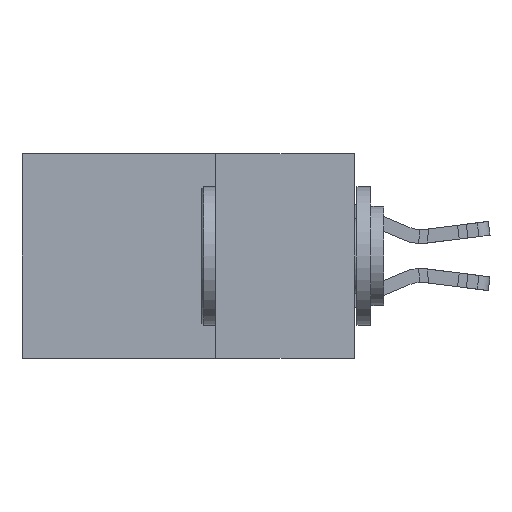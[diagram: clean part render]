
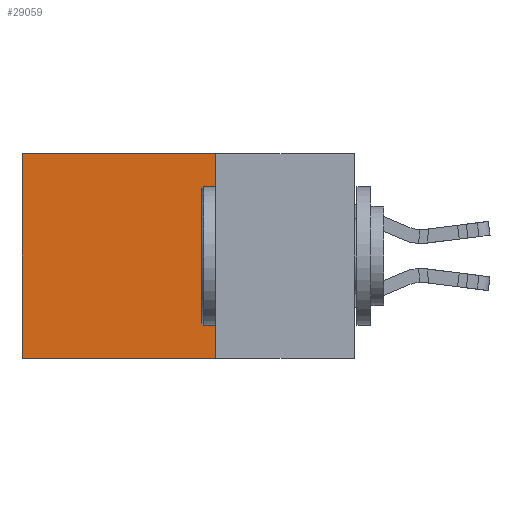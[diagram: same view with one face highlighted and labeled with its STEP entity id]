
A CAD part, left-side view. The second image highlights one B-rep face of the part: STEP entity #29059.
In plain terms, the highlighted planar face has unit normal (-1, 0, 0).
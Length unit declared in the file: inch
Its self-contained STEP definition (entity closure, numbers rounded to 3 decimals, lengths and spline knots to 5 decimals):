
#781 = CARTESIAN_POINT ( 'NONE',  ( 0.298, 0.25, 0. ) ) ;
#1526 = CARTESIAN_POINT ( 'NONE',  ( 0.298, 0.6, -0.37 ) ) ;
#2129 = DIRECTION ( 'NONE',  ( 0., 0., -1. ) ) ;
#2364 = CARTESIAN_POINT ( 'NONE',  ( 0.298, 0.6, 0. ) ) ;
#2925 = VERTEX_POINT ( 'NONE', #2364 ) ;
#3023 = VECTOR ( 'NONE', #2129, 39.37008 ) ;
#3134 = DIRECTION ( 'NONE',  ( 0., 0., -1. ) ) ;
#3246 = EDGE_LOOP ( 'NONE', ( #29673, #17705, #14978, #15695 ) ) ;
#3385 = DIRECTION ( 'NONE',  ( 0., 1., 0. ) ) ;
#3752 = EDGE_CURVE ( 'NONE', #8334, #28093, #27496, .T. ) ;
#4683 = EDGE_CURVE ( 'NONE', #2925, #28093, #22085, .T. ) ;
#4702 = CARTESIAN_POINT ( 'NONE',  ( 0.298, 0.25, 0. ) ) ;
#5238 = VECTOR ( 'NONE', #21957, 39.37008 ) ;
#7066 = DIRECTION ( 'NONE',  ( 0., 0., -1. ) ) ;
#8334 = VERTEX_POINT ( 'NONE', #19008 ) ;
#10009 = AXIS2_PLACEMENT_3D ( 'NONE', #781, #16998, #3134 ) ;
#13621 = EDGE_CURVE ( 'NONE', #26860, #2925, #23520, .T. ) ;
#13802 = FACE_OUTER_BOUND ( 'NONE', #3246, .T. ) ;
#13952 = EDGE_CURVE ( 'NONE', #26860, #8334, #26380, .T. ) ;
#14310 = VECTOR ( 'NONE', #7066, 39.37008 ) ;
#14978 = ORIENTED_EDGE ( 'NONE', *, *, #13952, .F. ) ;
#15695 = ORIENTED_EDGE ( 'NONE', *, *, #13621, .T. ) ;
#16998 = DIRECTION ( 'NONE',  ( 1., 0., 0. ) ) ;
#17705 = ORIENTED_EDGE ( 'NONE', *, *, #3752, .F. ) ;
#18091 = CARTESIAN_POINT ( 'NONE',  ( 0.298, 0.25, 0. ) ) ;
#19008 = CARTESIAN_POINT ( 'NONE',  ( 0.298, 0.25, -0.37 ) ) ;
#19715 = CARTESIAN_POINT ( 'NONE',  ( 0.298, 0.25, 0. ) ) ;
#21957 = DIRECTION ( 'NONE',  ( 0., 1., 0. ) ) ;
#22085 = LINE ( 'NONE', #22618, #3023 ) ;
#22618 = CARTESIAN_POINT ( 'NONE',  ( 0.298, 0.6, 0. ) ) ;
#23520 = LINE ( 'NONE', #19715, #5238 ) ;
#23563 = VECTOR ( 'NONE', #3385, 39.37008 ) ;
#26034 = PLANE ( 'NONE',  #10009 ) ;
#26380 = LINE ( 'NONE', #4702, #14310 ) ;
#26860 = VERTEX_POINT ( 'NONE', #18091 ) ;
#27496 = LINE ( 'NONE', #28211, #23563 ) ;
#28093 = VERTEX_POINT ( 'NONE', #1526 ) ;
#28211 = CARTESIAN_POINT ( 'NONE',  ( 0.298, 0.25, -0.37 ) ) ;
#29059 = ADVANCED_FACE ( 'NONE', ( #13802 ), #26034, .F. ) ;
#29673 = ORIENTED_EDGE ( 'NONE', *, *, #4683, .T. ) ;
